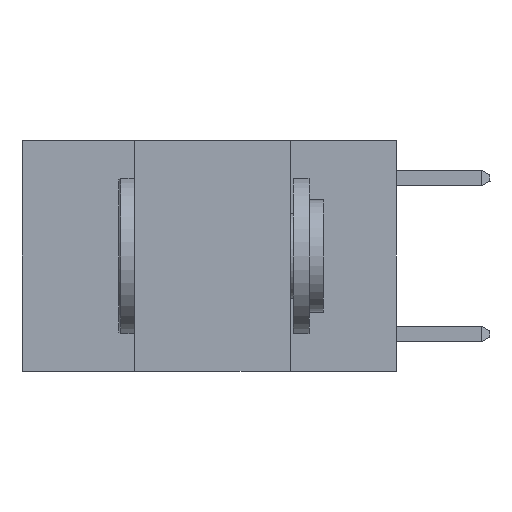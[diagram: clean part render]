
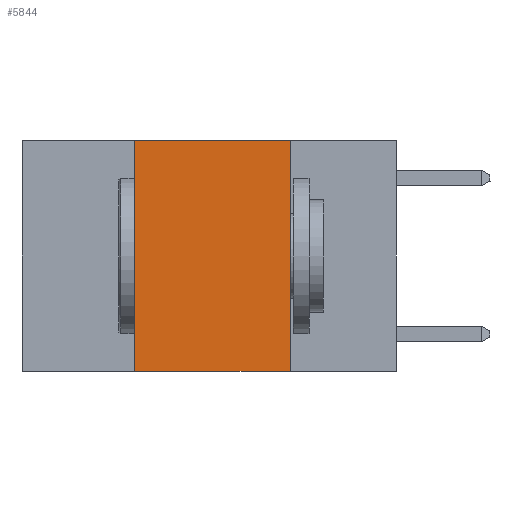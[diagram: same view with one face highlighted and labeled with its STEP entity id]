
A CAD part, left-side view. The second image highlights one B-rep face of the part: STEP entity #5844.
In plain terms, the highlighted planar face has unit normal (-1, 0, 0).
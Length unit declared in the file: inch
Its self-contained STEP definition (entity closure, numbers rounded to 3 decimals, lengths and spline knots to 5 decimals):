
#588 = DIRECTION ( 'NONE',  ( 0., 0., 1. ) ) ;
#617 = CARTESIAN_POINT ( 'NONE',  ( 0., 0.6, 0. ) ) ;
#854 = VERTEX_POINT ( 'NONE', #13984 ) ;
#1697 = CARTESIAN_POINT ( 'NONE',  ( 0., 0.17, 0. ) ) ;
#1924 = CARTESIAN_POINT ( 'NONE',  ( 0., 0.6, -0.37 ) ) ;
#1972 = ORIENTED_EDGE ( 'NONE', *, *, #4458, .F. ) ;
#2257 = VERTEX_POINT ( 'NONE', #6441 ) ;
#2703 = FACE_OUTER_BOUND ( 'NONE', #4828, .T. ) ;
#2997 = EDGE_CURVE ( 'NONE', #10184, #854, #8191, .T. ) ;
#3031 = VECTOR ( 'NONE', #12819, 39.37008 ) ;
#3090 = VECTOR ( 'NONE', #7171, 39.37008 ) ;
#3704 = LINE ( 'NONE', #1697, #3090 ) ;
#3790 = VECTOR ( 'NONE', #13657, 39.37008 ) ;
#4398 = EDGE_CURVE ( 'NONE', #2257, #854, #3704, .T. ) ;
#4458 = EDGE_CURVE ( 'NONE', #8194, #2257, #9401, .T. ) ;
#4828 = EDGE_LOOP ( 'NONE', ( #13428, #1972, #12854, #6791 ) ) ;
#5844 = ADVANCED_FACE ( 'NONE', ( #2703 ), #11357, .F. ) ;
#6441 = CARTESIAN_POINT ( 'NONE',  ( 0., 0.17, 0. ) ) ;
#6791 = ORIENTED_EDGE ( 'NONE', *, *, #2997, .T. ) ;
#7032 = DIRECTION ( 'NONE',  ( 0., 0., -1. ) ) ;
#7138 = CARTESIAN_POINT ( 'NONE',  ( 0., 0.42, 0. ) ) ;
#7171 = DIRECTION ( 'NONE',  ( 0., 0., -1. ) ) ;
#7239 = CARTESIAN_POINT ( 'NONE',  ( 0., 0.6, 0. ) ) ;
#7737 = CARTESIAN_POINT ( 'NONE',  ( 0., 0.42, 0. ) ) ;
#8191 = LINE ( 'NONE', #1924, #3031 ) ;
#8194 = VERTEX_POINT ( 'NONE', #7737 ) ;
#8210 = CARTESIAN_POINT ( 'NONE',  ( 0., 0.42, -0.37 ) ) ;
#8291 = LINE ( 'NONE', #7138, #12570 ) ;
#9392 = AXIS2_PLACEMENT_3D ( 'NONE', #7239, #11635, #7032 ) ;
#9401 = LINE ( 'NONE', #617, #3790 ) ;
#10184 = VERTEX_POINT ( 'NONE', #8210 ) ;
#11357 = PLANE ( 'NONE',  #9392 ) ;
#11586 = EDGE_CURVE ( 'NONE', #10184, #8194, #8291, .T. ) ;
#11635 = DIRECTION ( 'NONE',  ( 1., 0., 0. ) ) ;
#12570 = VECTOR ( 'NONE', #588, 39.37008 ) ;
#12819 = DIRECTION ( 'NONE',  ( 0., -1., 0. ) ) ;
#12854 = ORIENTED_EDGE ( 'NONE', *, *, #11586, .F. ) ;
#13428 = ORIENTED_EDGE ( 'NONE', *, *, #4398, .F. ) ;
#13657 = DIRECTION ( 'NONE',  ( 0., -1., 0. ) ) ;
#13984 = CARTESIAN_POINT ( 'NONE',  ( 0., 0.17, -0.37 ) ) ;
